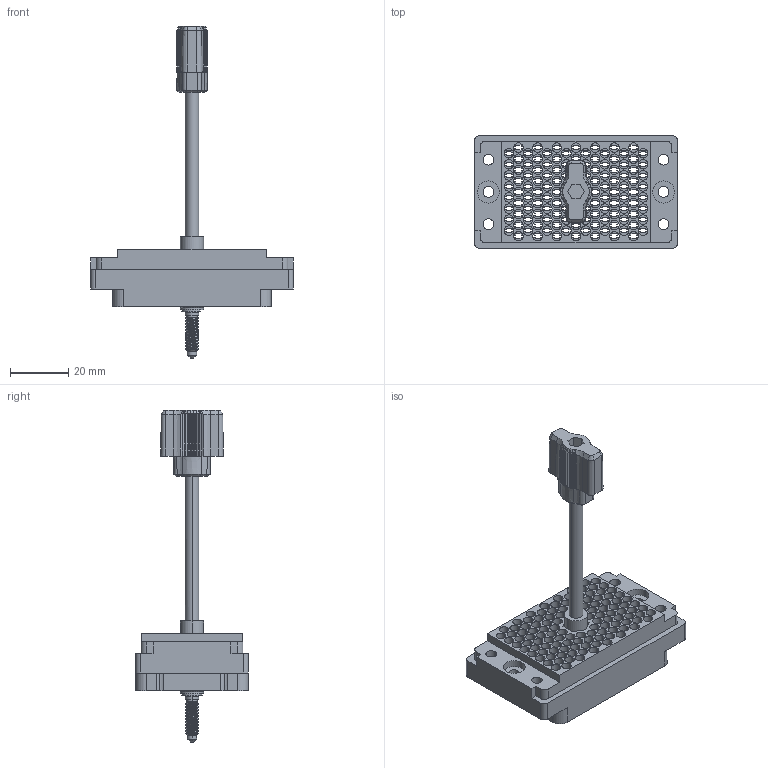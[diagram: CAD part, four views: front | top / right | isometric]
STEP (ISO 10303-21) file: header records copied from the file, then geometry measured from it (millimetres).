
FILE_DESCRIPTION (( 'STEP AP203' ), '1' );
FILE_NAME ('516-120-000-305.STEP', '2020-03-11T11:08:38', ( '' ), ( '' ), 'SwSTEP 2.0', 'SolidWorks 2016', '' );
FILE_SCHEMA (( 'CONFIG_CONTROL_DESIGN' ));
Length unit declared in the file: inch
Products named in the file (9): Actuating Screw Assy 090-120; 516-250-091-111; 516-253-190-107; Grub Screw; 516-120-000-305; 516 Plug Insulator_120; 516-253-095-100; 516-251-095-100; 516-254-091-109
Assembly tree (9 placements, depth 3):
  516-120-000-305
    516 Plug Insulator_120
    Actuating Screw Assy 090-120
      516-251-095-100
      516-254-091-109
      516-253-095-100  x2
      516-253-190-107
      516-250-091-111
      Grub Screw
Bounding box: 69.85 x 38.73 x 114.34 mm (x, y, z)
Volume: 24281.5 mm3; surface area: 31346.5 mm2
Topology: 8 solids, 8 shells, 2681 faces, 7851 edges, 5206 vertices
Faces by surface type: plane 1911, cylinder 691, cone 62, bspline 17
Entity records: 96874 total; most frequent: CARTESIAN_POINT 23015, ORIENTED_EDGE 15678, DIRECTION 14849, EDGE_CURVE 7839, VECTOR 5777, LINE 5777, VERTEX_POINT 5198, AXIS2_PLACEMENT_3D 4536
